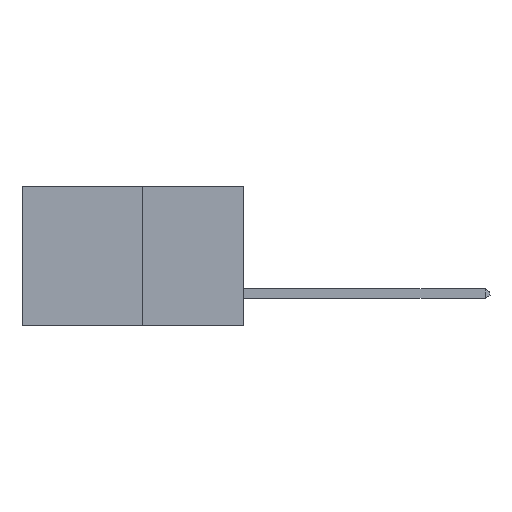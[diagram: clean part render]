
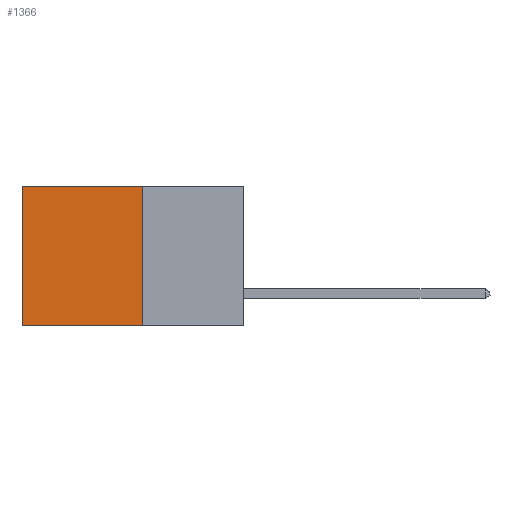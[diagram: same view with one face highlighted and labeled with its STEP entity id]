
A CAD part, left-side view. The second image highlights one B-rep face of the part: STEP entity #1366.
In plain terms, the highlighted planar face has unit normal (-1, 0, 0).
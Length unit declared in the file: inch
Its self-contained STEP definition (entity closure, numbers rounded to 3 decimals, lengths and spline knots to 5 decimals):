
#172 = EDGE_CURVE ( 'NONE', #3700, #6702, #5250, .T. ) ;
#693 = CARTESIAN_POINT ( 'NONE',  ( 0.277, 0.27, -0.37 ) ) ;
#1366 = ADVANCED_FACE ( 'NONE', ( #2717 ), #4853, .F. ) ;
#1380 = CARTESIAN_POINT ( 'NONE',  ( 0.277, 0.59, -0.37 ) ) ;
#2081 = CARTESIAN_POINT ( 'NONE',  ( 0.277, 0.27, -0.37 ) ) ;
#2262 = DIRECTION ( 'NONE',  ( 0., 0., -1. ) ) ;
#2375 = EDGE_CURVE ( 'NONE', #3235, #9385, #4158, .T. ) ;
#2717 = FACE_OUTER_BOUND ( 'NONE', #3873, .T. ) ;
#3235 = VERTEX_POINT ( 'NONE', #8487 ) ;
#3557 = CARTESIAN_POINT ( 'NONE',  ( 0.277, 0.27, 0. ) ) ;
#3700 = VERTEX_POINT ( 'NONE', #3557 ) ;
#3873 = EDGE_LOOP ( 'NONE', ( #7418, #4896, #10523, #5330 ) ) ;
#4158 = LINE ( 'NONE', #693, #8372 ) ;
#4357 = AXIS2_PLACEMENT_3D ( 'NONE', #5483, #5692, #5611 ) ;
#4447 = DIRECTION ( 'NONE',  ( 0., 1., 0. ) ) ;
#4853 = PLANE ( 'NONE',  #4357 ) ;
#4896 = ORIENTED_EDGE ( 'NONE', *, *, #2375, .F. ) ;
#4902 = VECTOR ( 'NONE', #2262, 39.37008 ) ;
#5178 = CARTESIAN_POINT ( 'NONE',  ( 0.277, 0.59, 0. ) ) ;
#5250 = LINE ( 'NONE', #8406, #9473 ) ;
#5330 = ORIENTED_EDGE ( 'NONE', *, *, #172, .T. ) ;
#5483 = CARTESIAN_POINT ( 'NONE',  ( 0.277, 0.27, -0.37 ) ) ;
#5611 = DIRECTION ( 'NONE',  ( 0., 0., -1. ) ) ;
#5692 = DIRECTION ( 'NONE',  ( 1., 0., 0. ) ) ;
#6702 = VERTEX_POINT ( 'NONE', #5178 ) ;
#6741 = LINE ( 'NONE', #2081, #8998 ) ;
#7151 = LINE ( 'NONE', #1380, #4902 ) ;
#7154 = DIRECTION ( 'NONE',  ( 0., 0., -1. ) ) ;
#7418 = ORIENTED_EDGE ( 'NONE', *, *, #10037, .T. ) ;
#7628 = EDGE_CURVE ( 'NONE', #3700, #3235, #6741, .T. ) ;
#8372 = VECTOR ( 'NONE', #10808, 39.37008 ) ;
#8406 = CARTESIAN_POINT ( 'NONE',  ( 0.277, 0.27, 0. ) ) ;
#8487 = CARTESIAN_POINT ( 'NONE',  ( 0.277, 0.27, -0.37 ) ) ;
#8998 = VECTOR ( 'NONE', #7154, 39.37008 ) ;
#9006 = CARTESIAN_POINT ( 'NONE',  ( 0.277, 0.59, -0.37 ) ) ;
#9385 = VERTEX_POINT ( 'NONE', #9006 ) ;
#9473 = VECTOR ( 'NONE', #4447, 39.37008 ) ;
#10037 = EDGE_CURVE ( 'NONE', #6702, #9385, #7151, .T. ) ;
#10523 = ORIENTED_EDGE ( 'NONE', *, *, #7628, .F. ) ;
#10808 = DIRECTION ( 'NONE',  ( 0., 1., 0. ) ) ;
